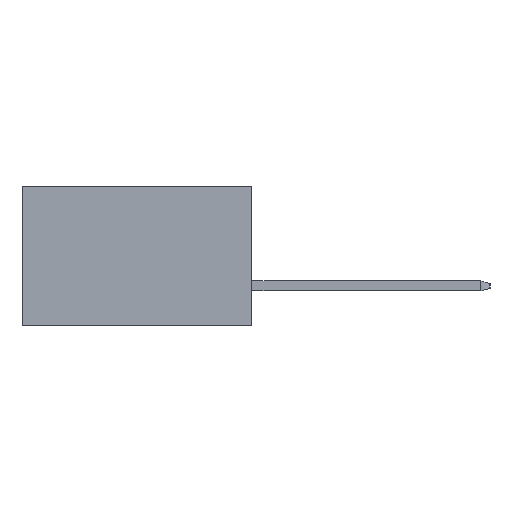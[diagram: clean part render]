
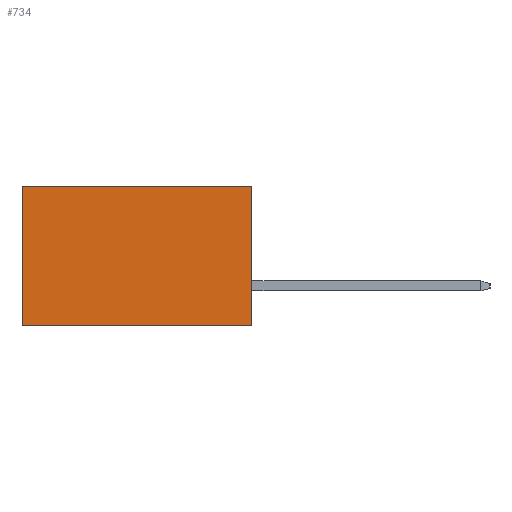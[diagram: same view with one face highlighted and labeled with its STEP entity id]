
A CAD part, left-side view. The second image highlights one B-rep face of the part: STEP entity #734.
In plain terms, the highlighted planar face has unit normal (-1, 0, 0).
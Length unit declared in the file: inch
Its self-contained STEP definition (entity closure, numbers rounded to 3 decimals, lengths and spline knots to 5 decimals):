
#102 = DIRECTION ( 'NONE',  ( 0., 1., 0. ) ) ;
#247 = LINE ( 'NONE', #5639, #1135 ) ;
#734 = ADVANCED_FACE ( 'NONE', ( #2347 ), #2391, .F. ) ;
#1135 = VECTOR ( 'NONE', #1954, 39.37008 ) ;
#1954 = DIRECTION ( 'NONE',  ( 0., 0., -1. ) ) ;
#2347 = FACE_OUTER_BOUND ( 'NONE', #3444, .T. ) ;
#2391 = PLANE ( 'NONE',  #2447 ) ;
#2442 = ORIENTED_EDGE ( 'NONE', *, *, #3187, .F. ) ;
#2447 = AXIS2_PLACEMENT_3D ( 'NONE', #5318, #9187, #8355 ) ;
#3187 = EDGE_CURVE ( 'NONE', #6752, #4346, #247, .T. ) ;
#3276 = DIRECTION ( 'NONE',  ( 0., 1., 0. ) ) ;
#3367 = LINE ( 'NONE', #4105, #4006 ) ;
#3444 = EDGE_LOOP ( 'NONE', ( #5550, #4666, #2442, #9510 ) ) ;
#3952 = EDGE_CURVE ( 'NONE', #5490, #5730, #5468, .T. ) ;
#4006 = VECTOR ( 'NONE', #3276, 39.37008 ) ;
#4018 = EDGE_CURVE ( 'NONE', #4346, #5730, #3367, .T. ) ;
#4105 = CARTESIAN_POINT ( 'NONE',  ( 0.3205, 0., -0.437 ) ) ;
#4254 = VECTOR ( 'NONE', #102, 39.37008 ) ;
#4346 = VERTEX_POINT ( 'NONE', #7491 ) ;
#4380 = EDGE_CURVE ( 'NONE', #6752, #5490, #6915, .T. ) ;
#4666 = ORIENTED_EDGE ( 'NONE', *, *, #4018, .F. ) ;
#5155 = CARTESIAN_POINT ( 'NONE',  ( 0.3205, 0.72, 0. ) ) ;
#5318 = CARTESIAN_POINT ( 'NONE',  ( 0.3205, 0., -0.437 ) ) ;
#5468 = LINE ( 'NONE', #8501, #7508 ) ;
#5490 = VERTEX_POINT ( 'NONE', #5155 ) ;
#5550 = ORIENTED_EDGE ( 'NONE', *, *, #3952, .T. ) ;
#5639 = CARTESIAN_POINT ( 'NONE',  ( 0.3205, 0., -0.437 ) ) ;
#5671 = CARTESIAN_POINT ( 'NONE',  ( 0.3205, 0., 0. ) ) ;
#5730 = VERTEX_POINT ( 'NONE', #7054 ) ;
#6752 = VERTEX_POINT ( 'NONE', #5671 ) ;
#6915 = LINE ( 'NONE', #8236, #4254 ) ;
#7054 = CARTESIAN_POINT ( 'NONE',  ( 0.3205, 0.72, -0.437 ) ) ;
#7491 = CARTESIAN_POINT ( 'NONE',  ( 0.3205, 0., -0.437 ) ) ;
#7508 = VECTOR ( 'NONE', #9181, 39.37008 ) ;
#8236 = CARTESIAN_POINT ( 'NONE',  ( 0.3205, 0., 0. ) ) ;
#8355 = DIRECTION ( 'NONE',  ( 0., 0., -1. ) ) ;
#8501 = CARTESIAN_POINT ( 'NONE',  ( 0.3205, 0.72, -0.437 ) ) ;
#9181 = DIRECTION ( 'NONE',  ( 0., 0., -1. ) ) ;
#9187 = DIRECTION ( 'NONE',  ( 1., 0., 0. ) ) ;
#9510 = ORIENTED_EDGE ( 'NONE', *, *, #4380, .T. ) ;
